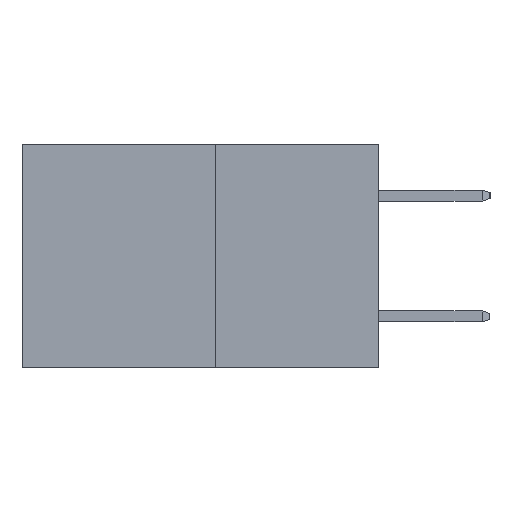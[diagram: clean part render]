
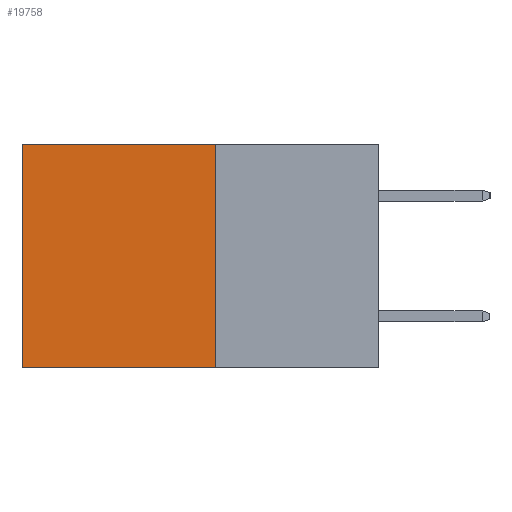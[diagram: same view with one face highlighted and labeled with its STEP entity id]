
A CAD part, left-side view. The second image highlights one B-rep face of the part: STEP entity #19758.
In plain terms, the highlighted planar face has unit normal (-1, 0, 0).
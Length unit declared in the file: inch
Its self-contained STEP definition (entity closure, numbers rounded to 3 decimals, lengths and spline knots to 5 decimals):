
#614 = CARTESIAN_POINT ( 'NONE',  ( 0.277, 0.59, -0.37 ) ) ;
#861 = VECTOR ( 'NONE', #6058, 39.37008 ) ;
#1363 = FACE_OUTER_BOUND ( 'NONE', #16197, .T. ) ;
#1798 = CARTESIAN_POINT ( 'NONE',  ( 0.277, 0.27, -0.37 ) ) ;
#1896 = VERTEX_POINT ( 'NONE', #15177 ) ;
#2313 = PLANE ( 'NONE',  #4527 ) ;
#4067 = CARTESIAN_POINT ( 'NONE',  ( 0.277, 0.27, 0. ) ) ;
#4223 = DIRECTION ( 'NONE',  ( 0., 0., -1. ) ) ;
#4243 = DIRECTION ( 'NONE',  ( 0., 0., -1. ) ) ;
#4527 = AXIS2_PLACEMENT_3D ( 'NONE', #7718, #14431, #4223 ) ;
#6058 = DIRECTION ( 'NONE',  ( 0., 0., -1. ) ) ;
#6638 = ORIENTED_EDGE ( 'NONE', *, *, #11918, .T. ) ;
#7718 = CARTESIAN_POINT ( 'NONE',  ( 0.277, 0.27, -0.37 ) ) ;
#8725 = CARTESIAN_POINT ( 'NONE',  ( 0.277, 0.27, -0.37 ) ) ;
#9456 = VECTOR ( 'NONE', #4243, 39.37008 ) ;
#9896 = LINE ( 'NONE', #8725, #18122 ) ;
#10430 = DIRECTION ( 'NONE',  ( 0., 1., 0. ) ) ;
#11501 = CARTESIAN_POINT ( 'NONE',  ( 0.277, 0.59, -0.37 ) ) ;
#11918 = EDGE_CURVE ( 'NONE', #13721, #1896, #21215, .T. ) ;
#12558 = VERTEX_POINT ( 'NONE', #1798 ) ;
#13057 = EDGE_CURVE ( 'NONE', #1896, #18068, #18216, .T. ) ;
#13467 = CARTESIAN_POINT ( 'NONE',  ( 0.277, 0.27, 0. ) ) ;
#13541 = DIRECTION ( 'NONE',  ( 0., 1., 0. ) ) ;
#13721 = VERTEX_POINT ( 'NONE', #4067 ) ;
#14431 = DIRECTION ( 'NONE',  ( 1., 0., 0. ) ) ;
#14470 = CARTESIAN_POINT ( 'NONE',  ( 0.277, 0.27, -0.37 ) ) ;
#14535 = ORIENTED_EDGE ( 'NONE', *, *, #20875, .F. ) ;
#15177 = CARTESIAN_POINT ( 'NONE',  ( 0.277, 0.59, 0. ) ) ;
#16197 = EDGE_LOOP ( 'NONE', ( #17859, #14535, #18867, #6638 ) ) ;
#16244 = VECTOR ( 'NONE', #13541, 39.37008 ) ;
#17859 = ORIENTED_EDGE ( 'NONE', *, *, #13057, .T. ) ;
#17917 = EDGE_CURVE ( 'NONE', #13721, #12558, #18981, .T. ) ;
#18068 = VERTEX_POINT ( 'NONE', #11501 ) ;
#18122 = VECTOR ( 'NONE', #10430, 39.37008 ) ;
#18216 = LINE ( 'NONE', #614, #9456 ) ;
#18867 = ORIENTED_EDGE ( 'NONE', *, *, #17917, .F. ) ;
#18981 = LINE ( 'NONE', #14470, #861 ) ;
#19758 = ADVANCED_FACE ( 'NONE', ( #1363 ), #2313, .F. ) ;
#20875 = EDGE_CURVE ( 'NONE', #12558, #18068, #9896, .T. ) ;
#21215 = LINE ( 'NONE', #13467, #16244 ) ;
